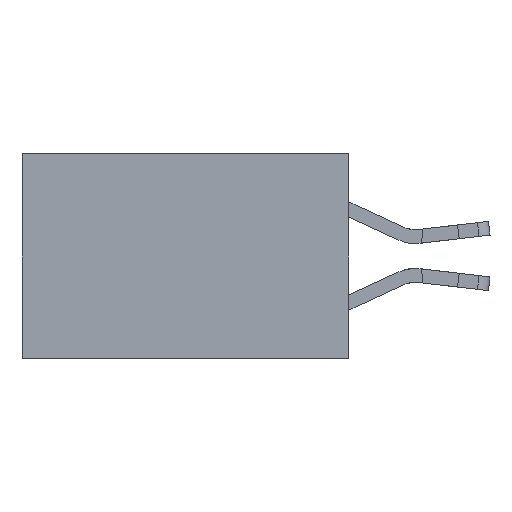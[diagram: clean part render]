
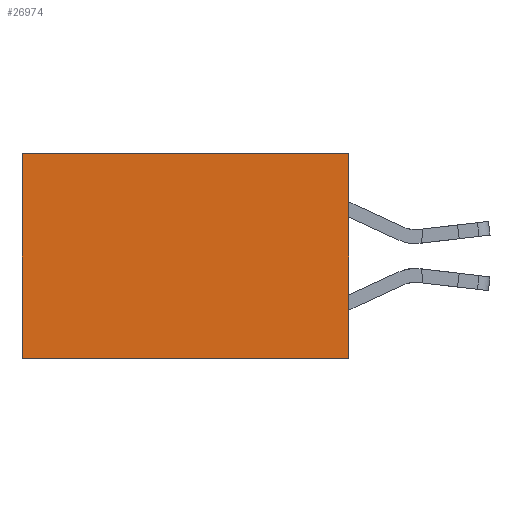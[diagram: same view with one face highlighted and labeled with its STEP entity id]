
A CAD part, left-side view. The second image highlights one B-rep face of the part: STEP entity #26974.
In plain terms, the highlighted planar face has unit normal (-1, 0, 0).
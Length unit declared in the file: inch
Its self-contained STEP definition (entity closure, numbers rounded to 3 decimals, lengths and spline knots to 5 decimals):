
#916 = ORIENTED_EDGE ( 'NONE', *, *, #22160, .T. ) ;
#1781 = DIRECTION ( 'NONE',  ( 0., 1., 0. ) ) ;
#3053 = VECTOR ( 'NONE', #13893, 39.37008 ) ;
#3346 = VERTEX_POINT ( 'NONE', #3932 ) ;
#3932 = CARTESIAN_POINT ( 'NONE',  ( 0.277, 0.59, -0.37 ) ) ;
#5418 = CARTESIAN_POINT ( 'NONE',  ( 0.277, 0.59, 0. ) ) ;
#6070 = ORIENTED_EDGE ( 'NONE', *, *, #23196, .F. ) ;
#7320 = CARTESIAN_POINT ( 'NONE',  ( 0.277, 0., -0.37 ) ) ;
#8288 = VERTEX_POINT ( 'NONE', #18694 ) ;
#9101 = CARTESIAN_POINT ( 'NONE',  ( 0.277, 0.59, -0.37 ) ) ;
#9486 = DIRECTION ( 'NONE',  ( 0., 0., -1. ) ) ;
#10431 = CARTESIAN_POINT ( 'NONE',  ( 0.277, 0., 0. ) ) ;
#10844 = CARTESIAN_POINT ( 'NONE',  ( 0.277, 0., 0. ) ) ;
#11688 = CARTESIAN_POINT ( 'NONE',  ( 0.277, 0., -0.37 ) ) ;
#11945 = DIRECTION ( 'NONE',  ( 0., 1., 0. ) ) ;
#11960 = VECTOR ( 'NONE', #11945, 39.37008 ) ;
#13893 = DIRECTION ( 'NONE',  ( 0., 0., -1. ) ) ;
#14313 = EDGE_CURVE ( 'NONE', #14739, #8288, #27404, .T. ) ;
#14739 = VERTEX_POINT ( 'NONE', #10844 ) ;
#14964 = VECTOR ( 'NONE', #19899, 39.37008 ) ;
#15921 = PLANE ( 'NONE',  #17745 ) ;
#16117 = VECTOR ( 'NONE', #1781, 39.37008 ) ;
#17745 = AXIS2_PLACEMENT_3D ( 'NONE', #7320, #22466, #9486 ) ;
#17784 = LINE ( 'NONE', #20604, #11960 ) ;
#18694 = CARTESIAN_POINT ( 'NONE',  ( 0.277, 0., -0.37 ) ) ;
#18895 = EDGE_LOOP ( 'NONE', ( #22841, #6070, #21483, #916 ) ) ;
#19098 = EDGE_CURVE ( 'NONE', #23945, #3346, #25774, .T. ) ;
#19899 = DIRECTION ( 'NONE',  ( 0., 0., -1. ) ) ;
#20604 = CARTESIAN_POINT ( 'NONE',  ( 0.277, 0., -0.37 ) ) ;
#21483 = ORIENTED_EDGE ( 'NONE', *, *, #14313, .F. ) ;
#22160 = EDGE_CURVE ( 'NONE', #14739, #23945, #22574, .T. ) ;
#22466 = DIRECTION ( 'NONE',  ( 1., 0., 0. ) ) ;
#22574 = LINE ( 'NONE', #10431, #16117 ) ;
#22841 = ORIENTED_EDGE ( 'NONE', *, *, #19098, .T. ) ;
#23196 = EDGE_CURVE ( 'NONE', #8288, #3346, #17784, .T. ) ;
#23945 = VERTEX_POINT ( 'NONE', #5418 ) ;
#25774 = LINE ( 'NONE', #9101, #14964 ) ;
#26916 = FACE_OUTER_BOUND ( 'NONE', #18895, .T. ) ;
#26974 = ADVANCED_FACE ( 'NONE', ( #26916 ), #15921, .F. ) ;
#27404 = LINE ( 'NONE', #11688, #3053 ) ;
